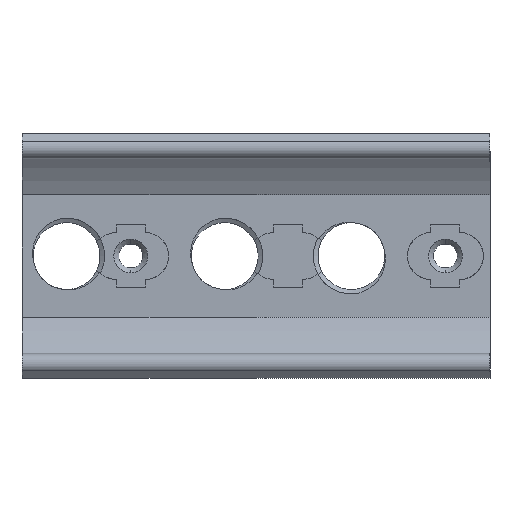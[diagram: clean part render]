
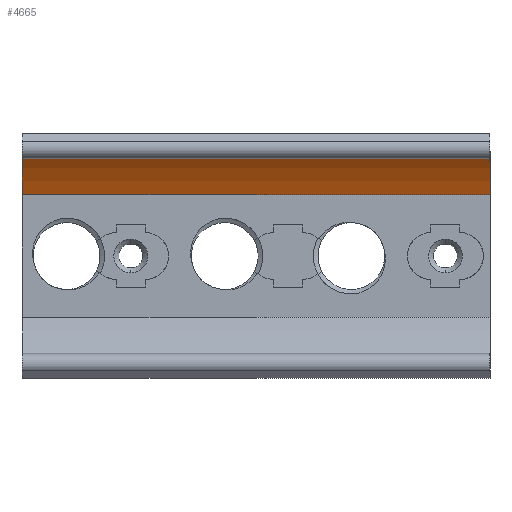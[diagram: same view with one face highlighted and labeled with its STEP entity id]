
A CAD part, top view. The second image highlights one B-rep face of the part: STEP entity #4665.
In plain terms, the highlighted cylindrical face has radius 20.32 mm (diameter 40.64 mm), a partial arc.
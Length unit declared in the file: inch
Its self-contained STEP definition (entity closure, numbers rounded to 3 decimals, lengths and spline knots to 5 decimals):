
#498 = AXIS2_PLACEMENT_3D ( 'NONE', #8339, #2139, #3099 ) ;
#1428 = ORIENTED_EDGE ( 'NONE', *, *, #4170, .F. ) ;
#1668 = DIRECTION ( 'NONE',  ( -1., 0., 0. ) ) ;
#1808 = DIRECTION ( 'NONE',  ( 0., -1., 0. ) ) ;
#2139 = DIRECTION ( 'NONE',  ( 1., 0., 0. ) ) ;
#2469 = VERTEX_POINT ( 'NONE', #11997 ) ;
#2787 = CARTESIAN_POINT ( 'NONE',  ( 1.47831, 0., 0.83854 ) ) ;
#3047 = DIRECTION ( 'NONE',  ( -1., 0., 0. ) ) ;
#3099 = DIRECTION ( 'NONE',  ( 0., 1., 0. ) ) ;
#3313 = EDGE_CURVE ( 'NONE', #7022, #2469, #12478, .T. ) ;
#3322 = VECTOR ( 'NONE', #3865, 39.37008 ) ;
#3865 = DIRECTION ( 'NONE',  ( 1., 0., 0. ) ) ;
#4170 = EDGE_CURVE ( 'NONE', #5727, #7022, #9582, .T. ) ;
#4665 = ADVANCED_FACE ( 'NONE', ( #5478 ), #5215, .F. ) ;
#5215 = CYLINDRICAL_SURFACE ( 'NONE', #9881, 0.8 ) ;
#5478 = FACE_OUTER_BOUND ( 'NONE', #6750, .T. ) ;
#5711 = CARTESIAN_POINT ( 'NONE',  ( 1.172, 0.3075, 0.1 ) ) ;
#5727 = VERTEX_POINT ( 'NONE', #5711 ) ;
#6102 = CARTESIAN_POINT ( 'NONE',  ( -1.182, 0.3075, 0.1 ) ) ;
#6397 = EDGE_CURVE ( 'NONE', #8040, #5727, #7574, .T. ) ;
#6412 = ORIENTED_EDGE ( 'NONE', *, *, #7379, .F. ) ;
#6750 = EDGE_LOOP ( 'NONE', ( #11947, #6412, #7423, #1428 ) ) ;
#7022 = VERTEX_POINT ( 'NONE', #9409 ) ;
#7379 = EDGE_CURVE ( 'NONE', #2469, #8040, #10458, .T. ) ;
#7423 = ORIENTED_EDGE ( 'NONE', *, *, #3313, .F. ) ;
#7574 = CIRCLE ( 'NONE', #8759, 0.8 ) ;
#8040 = VERTEX_POINT ( 'NONE', #10119 ) ;
#8339 = CARTESIAN_POINT ( 'NONE',  ( -1.172, 0., 0.83854 ) ) ;
#8759 = AXIS2_PLACEMENT_3D ( 'NONE', #10401, #3047, #12319 ) ;
#9204 = DIRECTION ( 'NONE',  ( -1., 0., 0. ) ) ;
#9409 = CARTESIAN_POINT ( 'NONE',  ( -1.172, 0.3075, 0.1 ) ) ;
#9582 = LINE ( 'NONE', #6102, #12012 ) ;
#9881 = AXIS2_PLACEMENT_3D ( 'NONE', #2787, #1668, #1808 ) ;
#9888 = CARTESIAN_POINT ( 'NONE',  ( -1.35162, 0.50058, 0.21451 ) ) ;
#10119 = CARTESIAN_POINT ( 'NONE',  ( 1.172, 0.50058, 0.21451 ) ) ;
#10401 = CARTESIAN_POINT ( 'NONE',  ( 1.172, 0., 0.83854 ) ) ;
#10458 = LINE ( 'NONE', #9888, #3322 ) ;
#11947 = ORIENTED_EDGE ( 'NONE', *, *, #6397, .F. ) ;
#11997 = CARTESIAN_POINT ( 'NONE',  ( -1.172, 0.50058, 0.21451 ) ) ;
#12012 = VECTOR ( 'NONE', #9204, 39.37008 ) ;
#12319 = DIRECTION ( 'NONE',  ( 0., -1., 0. ) ) ;
#12478 = CIRCLE ( 'NONE', #498, 0.8 ) ;
